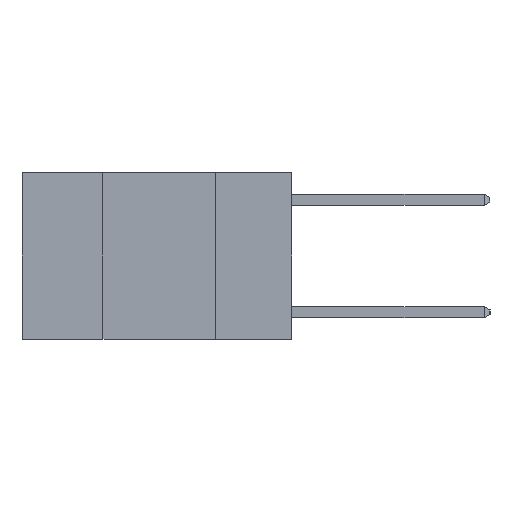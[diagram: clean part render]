
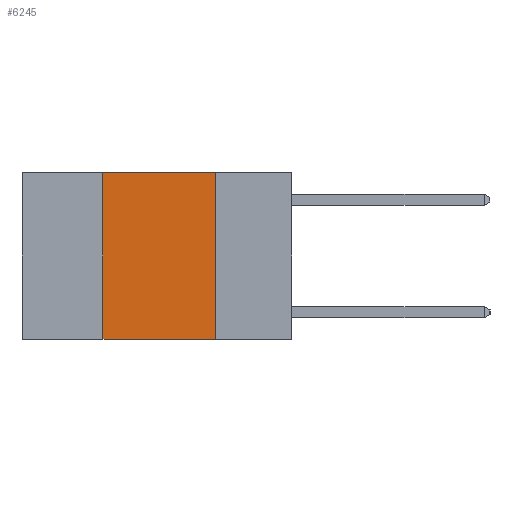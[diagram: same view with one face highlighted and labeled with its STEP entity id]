
A CAD part, left-side view. The second image highlights one B-rep face of the part: STEP entity #6245.
In plain terms, the highlighted planar face has unit normal (-1, 0, 0).
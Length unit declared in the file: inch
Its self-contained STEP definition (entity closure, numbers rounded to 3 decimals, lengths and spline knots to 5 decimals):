
#130 = FACE_OUTER_BOUND ( 'NONE', #6741, .T. ) ;
#350 = ORIENTED_EDGE ( 'NONE', *, *, #7101, .F. ) ;
#617 = VECTOR ( 'NONE', #1140, 39.37008 ) ;
#715 = ORIENTED_EDGE ( 'NONE', *, *, #6575, .F. ) ;
#1140 = DIRECTION ( 'NONE',  ( 0., 0., 1. ) ) ;
#1206 = CARTESIAN_POINT ( 'NONE',  ( 0., 0.17, -0.37 ) ) ;
#2549 = DIRECTION ( 'NONE',  ( 0., 0., -1. ) ) ;
#2700 = VERTEX_POINT ( 'NONE', #8613 ) ;
#2770 = VERTEX_POINT ( 'NONE', #6370 ) ;
#3356 = CARTESIAN_POINT ( 'NONE',  ( 0., 0.6, -0.37 ) ) ;
#3468 = CARTESIAN_POINT ( 'NONE',  ( 0., 0.42, -0.37 ) ) ;
#3618 = DIRECTION ( 'NONE',  ( 0., -1., 0. ) ) ;
#4433 = VECTOR ( 'NONE', #3618, 39.37008 ) ;
#4582 = ORIENTED_EDGE ( 'NONE', *, *, #8475, .F. ) ;
#4642 = DIRECTION ( 'NONE',  ( 0., 0., -1. ) ) ;
#4856 = PLANE ( 'NONE',  #9289 ) ;
#6245 = ADVANCED_FACE ( 'NONE', ( #130 ), #4856, .F. ) ;
#6361 = CARTESIAN_POINT ( 'NONE',  ( 0., 0.6, 0. ) ) ;
#6370 = CARTESIAN_POINT ( 'NONE',  ( 0., 0.17, 0. ) ) ;
#6575 = EDGE_CURVE ( 'NONE', #2770, #9036, #7239, .T. ) ;
#6741 = EDGE_LOOP ( 'NONE', ( #715, #4582, #350, #7926 ) ) ;
#6756 = LINE ( 'NONE', #8059, #617 ) ;
#6994 = VECTOR ( 'NONE', #4642, 39.37008 ) ;
#7101 = EDGE_CURVE ( 'NONE', #9041, #2700, #6756, .T. ) ;
#7157 = DIRECTION ( 'NONE',  ( 1., 0., 0. ) ) ;
#7239 = LINE ( 'NONE', #9070, #6994 ) ;
#7341 = LINE ( 'NONE', #3356, #9375 ) ;
#7467 = CARTESIAN_POINT ( 'NONE',  ( 0., 0.6, 0. ) ) ;
#7699 = EDGE_CURVE ( 'NONE', #9041, #9036, #7341, .T. ) ;
#7926 = ORIENTED_EDGE ( 'NONE', *, *, #7699, .T. ) ;
#8059 = CARTESIAN_POINT ( 'NONE',  ( 0., 0.42, 0. ) ) ;
#8475 = EDGE_CURVE ( 'NONE', #2700, #2770, #8768, .T. ) ;
#8613 = CARTESIAN_POINT ( 'NONE',  ( 0., 0.42, 0. ) ) ;
#8759 = DIRECTION ( 'NONE',  ( 0., -1., 0. ) ) ;
#8768 = LINE ( 'NONE', #7467, #4433 ) ;
#9036 = VERTEX_POINT ( 'NONE', #1206 ) ;
#9041 = VERTEX_POINT ( 'NONE', #3468 ) ;
#9070 = CARTESIAN_POINT ( 'NONE',  ( 0., 0.17, 0. ) ) ;
#9289 = AXIS2_PLACEMENT_3D ( 'NONE', #6361, #7157, #2549 ) ;
#9375 = VECTOR ( 'NONE', #8759, 39.37008 ) ;
